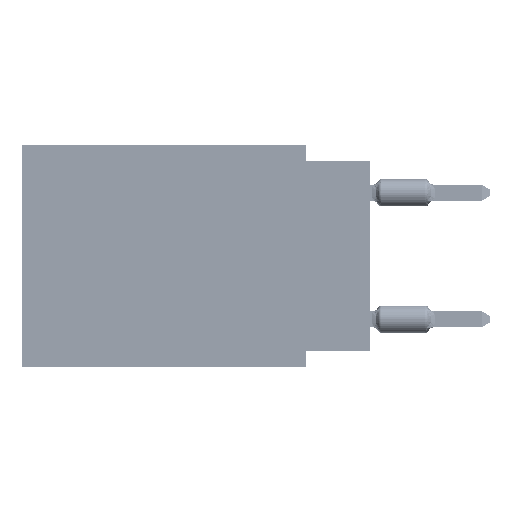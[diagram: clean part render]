
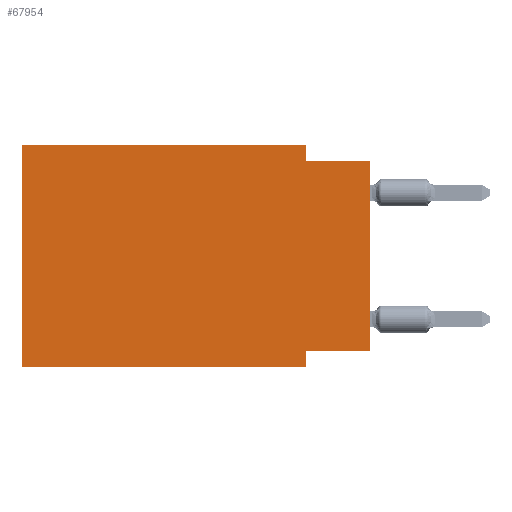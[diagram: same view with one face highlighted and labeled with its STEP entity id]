
A CAD part, left-side view. The second image highlights one B-rep face of the part: STEP entity #67954.
In plain terms, the highlighted planar face has unit normal (-1, 0, 0).
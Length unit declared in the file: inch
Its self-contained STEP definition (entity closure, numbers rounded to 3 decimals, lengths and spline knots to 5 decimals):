
#2454 = VERTEX_POINT ( 'NONE', #93174 ) ;
#4147 = DIRECTION ( 'NONE',  ( 0., 0., -1. ) ) ;
#8666 = CARTESIAN_POINT ( 'NONE',  ( 0., 0., -0.025 ) ) ;
#9237 = PLANE ( 'NONE',  #75784 ) ;
#11005 = ORIENTED_EDGE ( 'NONE', *, *, #82325, .F. ) ;
#11290 = CARTESIAN_POINT ( 'NONE',  ( 0., 0.1, -0.35 ) ) ;
#13856 = VERTEX_POINT ( 'NONE', #8666 ) ;
#14294 = EDGE_LOOP ( 'NONE', ( #104497, #30967, #19987, #105217, #11005, #39066, #79126, #21265 ) ) ;
#14712 = VECTOR ( 'NONE', #4147, 39.37008 ) ;
#14772 = CARTESIAN_POINT ( 'NONE',  ( 0., 0., -0.025 ) ) ;
#15385 = LINE ( 'NONE', #47648, #73975 ) ;
#15695 = CARTESIAN_POINT ( 'NONE',  ( 0., 0., -0.325 ) ) ;
#15899 = DIRECTION ( 'NONE',  ( 0., 1., 0. ) ) ;
#16270 = DIRECTION ( 'NONE',  ( 0., 0., 1. ) ) ;
#18686 = LINE ( 'NONE', #86372, #36666 ) ;
#18774 = CARTESIAN_POINT ( 'NONE',  ( 0., 0.1, 0. ) ) ;
#19987 = ORIENTED_EDGE ( 'NONE', *, *, #97393, .F. ) ;
#20280 = LINE ( 'NONE', #85830, #14712 ) ;
#21265 = ORIENTED_EDGE ( 'NONE', *, *, #95101, .F. ) ;
#21943 = VECTOR ( 'NONE', #72763, 39.37008 ) ;
#23001 = VECTOR ( 'NONE', #16270, 39.37008 ) ;
#23837 = CARTESIAN_POINT ( 'NONE',  ( 0., 0.55, -0.35 ) ) ;
#24149 = VERTEX_POINT ( 'NONE', #56931 ) ;
#25808 = VERTEX_POINT ( 'NONE', #54015 ) ;
#30298 = EDGE_CURVE ( 'NONE', #25808, #13856, #87853, .T. ) ;
#30967 = ORIENTED_EDGE ( 'NONE', *, *, #30298, .F. ) ;
#31450 = DIRECTION ( 'NONE',  ( 0., -1., 0. ) ) ;
#31996 = CARTESIAN_POINT ( 'NONE',  ( 0., 0.55, 0. ) ) ;
#32894 = DIRECTION ( 'NONE',  ( 0., 0., -1. ) ) ;
#33421 = DIRECTION ( 'NONE',  ( 1., 0., 0. ) ) ;
#34627 = EDGE_CURVE ( 'NONE', #35980, #2454, #81922, .T. ) ;
#35980 = VERTEX_POINT ( 'NONE', #31996 ) ;
#36570 = VECTOR ( 'NONE', #66075, 39.37008 ) ;
#36666 = VECTOR ( 'NONE', #52509, 39.37008 ) ;
#39066 = ORIENTED_EDGE ( 'NONE', *, *, #93735, .T. ) ;
#46355 = VERTEX_POINT ( 'NONE', #11290 ) ;
#47588 = CARTESIAN_POINT ( 'NONE',  ( 0., 0.55, 0. ) ) ;
#47648 = CARTESIAN_POINT ( 'NONE',  ( 0., 0., -0.325 ) ) ;
#49984 = VECTOR ( 'NONE', #104995, 39.37008 ) ;
#52509 = DIRECTION ( 'NONE',  ( 0., 0., 1. ) ) ;
#54015 = CARTESIAN_POINT ( 'NONE',  ( 0., 0.1, -0.025 ) ) ;
#56256 = VERTEX_POINT ( 'NONE', #15695 ) ;
#56931 = CARTESIAN_POINT ( 'NONE',  ( 0., 0.55, -0.35 ) ) ;
#66075 = DIRECTION ( 'NONE',  ( 0., 0., -1. ) ) ;
#67954 = ADVANCED_FACE ( 'NONE', ( #99524 ), #9237, .F. ) ;
#72763 = DIRECTION ( 'NONE',  ( 0., -1., 0. ) ) ;
#73975 = VECTOR ( 'NONE', #15899, 39.37008 ) ;
#74583 = VERTEX_POINT ( 'NONE', #104258 ) ;
#75784 = AXIS2_PLACEMENT_3D ( 'NONE', #82311, #33421, #32894 ) ;
#79126 = ORIENTED_EDGE ( 'NONE', *, *, #100524, .F. ) ;
#81922 = LINE ( 'NONE', #47588, #91239 ) ;
#82311 = CARTESIAN_POINT ( 'NONE',  ( 0., 0.55, 0. ) ) ;
#82325 = EDGE_CURVE ( 'NONE', #24149, #35980, #18686, .T. ) ;
#83260 = LINE ( 'NONE', #18774, #36570 ) ;
#85830 = CARTESIAN_POINT ( 'NONE',  ( 0., 0.1, -0.35 ) ) ;
#86372 = CARTESIAN_POINT ( 'NONE',  ( 0., 0.55, 0. ) ) ;
#87853 = LINE ( 'NONE', #14772, #21943 ) ;
#89897 = CARTESIAN_POINT ( 'NONE',  ( 0., 0., 0. ) ) ;
#91239 = VECTOR ( 'NONE', #31450, 39.37008 ) ;
#93174 = CARTESIAN_POINT ( 'NONE',  ( 0., 0.1, 0. ) ) ;
#93735 = EDGE_CURVE ( 'NONE', #24149, #46355, #96926, .T. ) ;
#95101 = EDGE_CURVE ( 'NONE', #56256, #74583, #15385, .T. ) ;
#96926 = LINE ( 'NONE', #23837, #49984 ) ;
#97393 = EDGE_CURVE ( 'NONE', #2454, #25808, #83260, .T. ) ;
#97977 = LINE ( 'NONE', #89897, #23001 ) ;
#98121 = EDGE_CURVE ( 'NONE', #56256, #13856, #97977, .T. ) ;
#99524 = FACE_OUTER_BOUND ( 'NONE', #14294, .T. ) ;
#100524 = EDGE_CURVE ( 'NONE', #74583, #46355, #20280, .T. ) ;
#104258 = CARTESIAN_POINT ( 'NONE',  ( 0., 0.1, -0.325 ) ) ;
#104497 = ORIENTED_EDGE ( 'NONE', *, *, #98121, .T. ) ;
#104995 = DIRECTION ( 'NONE',  ( 0., -1., 0. ) ) ;
#105217 = ORIENTED_EDGE ( 'NONE', *, *, #34627, .F. ) ;
